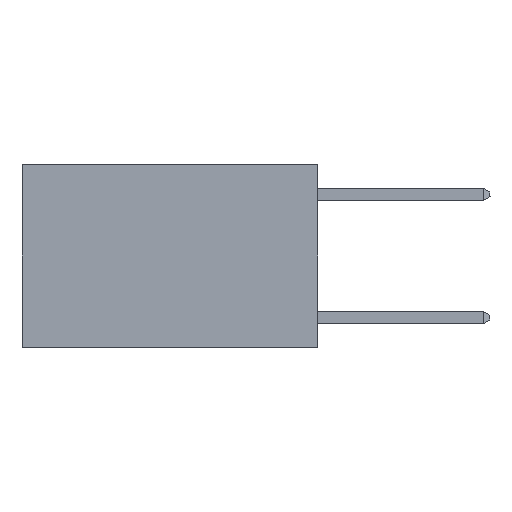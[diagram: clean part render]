
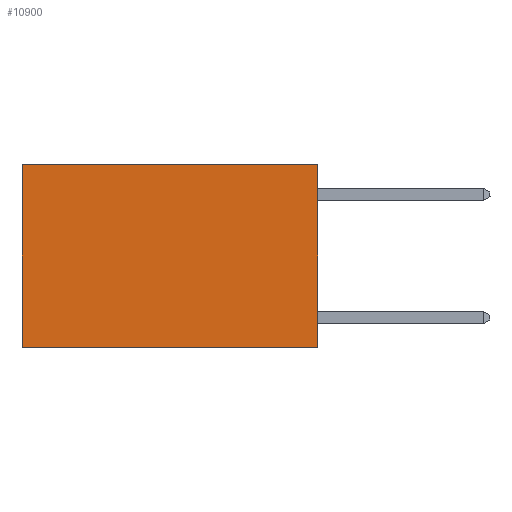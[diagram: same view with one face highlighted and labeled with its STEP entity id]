
A CAD part, left-side view. The second image highlights one B-rep face of the part: STEP entity #10900.
In plain terms, the highlighted planar face has unit normal (-1, 0, 0).
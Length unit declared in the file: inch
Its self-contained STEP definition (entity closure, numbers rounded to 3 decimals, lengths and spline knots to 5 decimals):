
#414 = CARTESIAN_POINT ( 'NONE',  ( 0.2625, 0., -0.37 ) ) ;
#796 = VERTEX_POINT ( 'NONE', #414 ) ;
#1789 = DIRECTION ( 'NONE',  ( 0., 1., 0. ) ) ;
#2450 = AXIS2_PLACEMENT_3D ( 'NONE', #3806, #4979, #13102 ) ;
#3529 = EDGE_CURVE ( 'NONE', #796, #9074, #7469, .T. ) ;
#3806 = CARTESIAN_POINT ( 'NONE',  ( 0.2625, 0., 0. ) ) ;
#4345 = CARTESIAN_POINT ( 'NONE',  ( 0.2625, 0., 0. ) ) ;
#4736 = VECTOR ( 'NONE', #1789, 39.37008 ) ;
#4979 = DIRECTION ( 'NONE',  ( 1., 0., 0. ) ) ;
#5761 = CARTESIAN_POINT ( 'NONE',  ( 0.2625, 0.6, 0. ) ) ;
#6946 = DIRECTION ( 'NONE',  ( 0., 0., -1. ) ) ;
#7019 = DIRECTION ( 'NONE',  ( 0., 1., 0. ) ) ;
#7469 = LINE ( 'NONE', #10027, #4736 ) ;
#7947 = CARTESIAN_POINT ( 'NONE',  ( 0.2625, 0., 0. ) ) ;
#8154 = CARTESIAN_POINT ( 'NONE',  ( 0.2625, 0., 0. ) ) ;
#8544 = EDGE_CURVE ( 'NONE', #9315, #796, #14035, .T. ) ;
#9062 = DIRECTION ( 'NONE',  ( 0., 0., -1. ) ) ;
#9074 = VERTEX_POINT ( 'NONE', #9881 ) ;
#9315 = VERTEX_POINT ( 'NONE', #7947 ) ;
#9468 = EDGE_CURVE ( 'NONE', #9315, #14184, #14360, .T. ) ;
#9881 = CARTESIAN_POINT ( 'NONE',  ( 0.2625, 0.6, -0.37 ) ) ;
#10027 = CARTESIAN_POINT ( 'NONE',  ( 0.2625, 0., -0.37 ) ) ;
#10156 = EDGE_LOOP ( 'NONE', ( #11632, #11727, #11749, #11868 ) ) ;
#10784 = PLANE ( 'NONE',  #2450 ) ;
#10857 = CARTESIAN_POINT ( 'NONE',  ( 0.2625, 0.6, 0. ) ) ;
#10900 = ADVANCED_FACE ( 'NONE', ( #13230 ), #10784, .F. ) ;
#10963 = VECTOR ( 'NONE', #9062, 39.37008 ) ;
#11298 = VECTOR ( 'NONE', #7019, 39.37008 ) ;
#11632 = ORIENTED_EDGE ( 'NONE', *, *, #14917, .T. ) ;
#11727 = ORIENTED_EDGE ( 'NONE', *, *, #3529, .F. ) ;
#11749 = ORIENTED_EDGE ( 'NONE', *, *, #8544, .F. ) ;
#11868 = ORIENTED_EDGE ( 'NONE', *, *, #9468, .T. ) ;
#12061 = LINE ( 'NONE', #5761, #14764 ) ;
#13102 = DIRECTION ( 'NONE',  ( 0., 0., -1. ) ) ;
#13230 = FACE_OUTER_BOUND ( 'NONE', #10156, .T. ) ;
#14035 = LINE ( 'NONE', #4345, #10963 ) ;
#14184 = VERTEX_POINT ( 'NONE', #10857 ) ;
#14360 = LINE ( 'NONE', #8154, #11298 ) ;
#14764 = VECTOR ( 'NONE', #6946, 39.37008 ) ;
#14917 = EDGE_CURVE ( 'NONE', #14184, #9074, #12061, .T. ) ;
